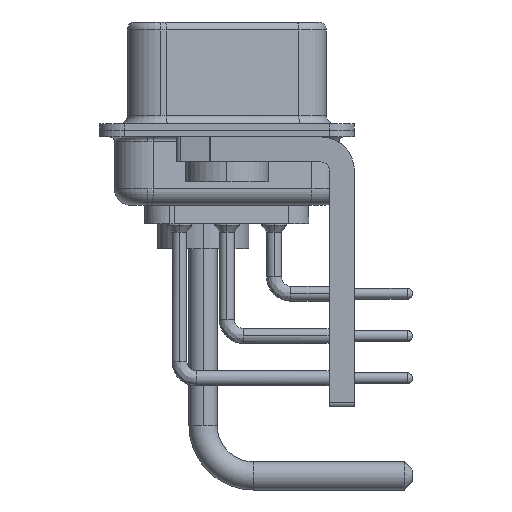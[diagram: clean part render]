
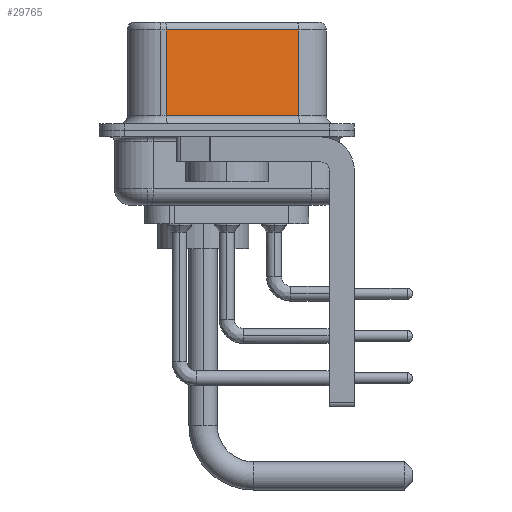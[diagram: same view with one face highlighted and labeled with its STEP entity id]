
A CAD part, left-side view. The second image highlights one B-rep face of the part: STEP entity #29765.
In plain terms, the highlighted planar face has unit normal (-0.985, -0.174, 0).
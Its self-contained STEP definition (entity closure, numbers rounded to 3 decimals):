
#1252 = FACE_OUTER_BOUND ( 'NONE', #18956, .T. ) ;
#1812 = CARTESIAN_POINT ( 'NONE',  ( 5.132, -4.322, 6.52 ) ) ;
#2247 = CARTESIAN_POINT ( 'NONE',  ( 3.73, 3.628, 6.52 ) ) ;
#2647 = VERTEX_POINT ( 'NONE', #19723 ) ;
#3743 = LINE ( 'NONE', #20869, #13269 ) ;
#4773 = CARTESIAN_POINT ( 'NONE',  ( 5.132, -4.322, 6.02 ) ) ;
#5268 = ORIENTED_EDGE ( 'NONE', *, *, #32233, .T. ) ;
#6297 = CARTESIAN_POINT ( 'NONE',  ( 5.132, -4.322, 0.9 ) ) ;
#7741 = ORIENTED_EDGE ( 'NONE', *, *, #36669, .F. ) ;
#8422 = DIRECTION ( 'NONE',  ( -0.174, 0.985, 0. ) ) ;
#11634 = VERTEX_POINT ( 'NONE', #25267 ) ;
#11768 = DIRECTION ( 'NONE',  ( 0.174, -0.985, 0. ) ) ;
#13110 = DIRECTION ( 'NONE',  ( -0.174, 0.985, 0. ) ) ;
#13269 = VECTOR ( 'NONE', #32138, 1000. ) ;
#13522 = AXIS2_PLACEMENT_3D ( 'NONE', #1812, #32845, #13110 ) ;
#13613 = ORIENTED_EDGE ( 'NONE', *, *, #18046, .T. ) ;
#14043 = CARTESIAN_POINT ( 'NONE',  ( 5.132, -4.322, 0.9 ) ) ;
#14844 = EDGE_CURVE ( 'NONE', #2647, #11634, #36489, .T. ) ;
#15599 = VECTOR ( 'NONE', #8422, 1000. ) ;
#18046 = EDGE_CURVE ( 'NONE', #30336, #2647, #34179, .T. ) ;
#18956 = EDGE_LOOP ( 'NONE', ( #7741, #13613, #33016, #5268 ) ) ;
#19699 = CARTESIAN_POINT ( 'NONE',  ( 5.132, -4.322, 6.02 ) ) ;
#19723 = CARTESIAN_POINT ( 'NONE',  ( 3.73, 3.628, 6.02 ) ) ;
#20869 = CARTESIAN_POINT ( 'NONE',  ( 5.132, -4.322, 6.52 ) ) ;
#22404 = VECTOR ( 'NONE', #22580, 1000. ) ;
#22580 = DIRECTION ( 'NONE',  ( 0., 0., -1. ) ) ;
#22706 = LINE ( 'NONE', #14043, #36500 ) ;
#25267 = CARTESIAN_POINT ( 'NONE',  ( 3.73, 3.628, 0.9 ) ) ;
#27595 = PLANE ( 'NONE',  #13522 ) ;
#29765 = ADVANCED_FACE ( 'NONE', ( #1252 ), #27595, .F. ) ;
#30336 = VERTEX_POINT ( 'NONE', #4773 ) ;
#32138 = DIRECTION ( 'NONE',  ( 0., 0., -1. ) ) ;
#32233 = EDGE_CURVE ( 'NONE', #11634, #34416, #22706, .T. ) ;
#32845 = DIRECTION ( 'NONE',  ( 0.985, 0.174, 0. ) ) ;
#33016 = ORIENTED_EDGE ( 'NONE', *, *, #14844, .T. ) ;
#34179 = LINE ( 'NONE', #19699, #15599 ) ;
#34416 = VERTEX_POINT ( 'NONE', #6297 ) ;
#36489 = LINE ( 'NONE', #2247, #22404 ) ;
#36500 = VECTOR ( 'NONE', #11768, 1000. ) ;
#36669 = EDGE_CURVE ( 'NONE', #30336, #34416, #3743, .T. ) ;
